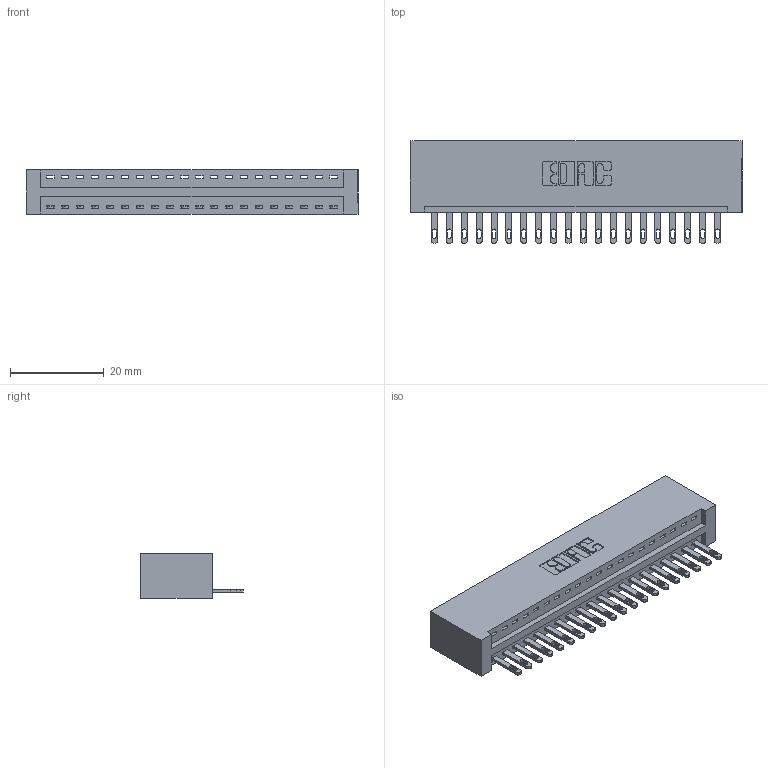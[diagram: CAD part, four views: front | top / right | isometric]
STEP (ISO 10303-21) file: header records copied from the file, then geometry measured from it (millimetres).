
FILE_DESCRIPTION (( 'STEP AP203' ), '1' );
FILE_NAME ('896-020-500-101.STEP', '2021-07-27T16:25:18', ( '' ), ( '' ), 'SwSTEP 2.0', 'SolidWorks 2020', '' );
FILE_SCHEMA (( 'CONFIG_CONTROL_DESIGN' ));
Length unit declared in the file: inch
Products named in the file (3): 846 Part_No Mounting Lugs; 345-292-001_345-293-100; 896-020-500-101
Assembly tree (21 placements, depth 2):
  896-020-500-101
    846 Part_No Mounting Lugs
    345-292-001_345-293-100  x20
Bounding box: 70.74 x 21.84 x 9.4 mm (x, y, z)
Volume: 7181.5 mm3; surface area: 8860.3 mm2
Topology: 21 solids, 21 shells, 1194 faces, 3665 edges, 2442 vertices
Faces by surface type: plane 752, cylinder 442
Entity records: 15027 total; most frequent: CARTESIAN_POINT 2588, ORIENTED_EDGE 2542, DIRECTION 2307, EDGE_CURVE 1271, VECTOR 1063, LINE 1063, VERTEX_POINT 846, AXIS2_PLACEMENT_3D 622
